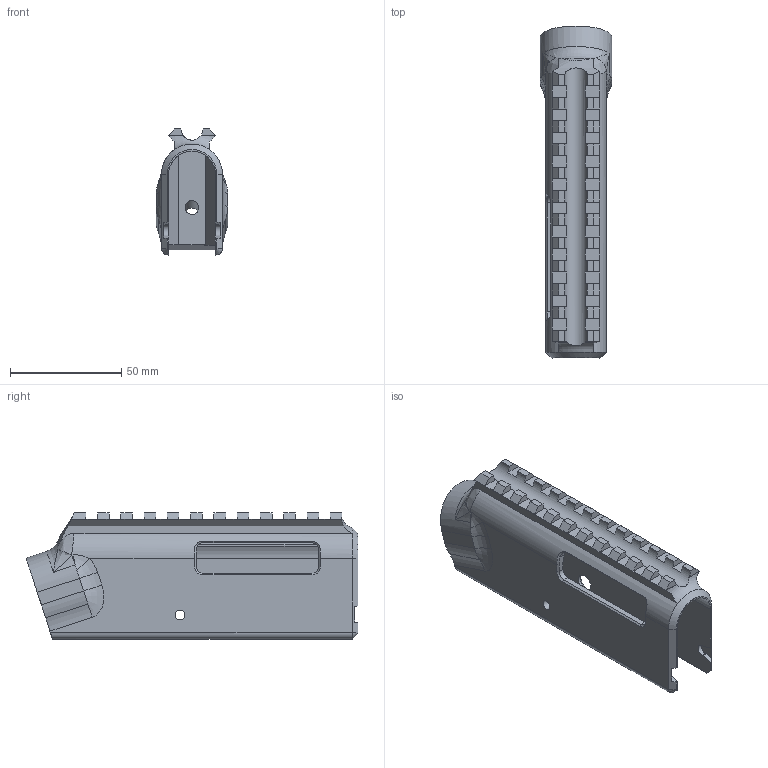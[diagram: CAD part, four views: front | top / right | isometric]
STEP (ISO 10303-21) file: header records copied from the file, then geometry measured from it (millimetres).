
FILE_DESCRIPTION(/* description */ (''),/* implementation_level */ '2;1');
FILE_NAME(/* name */ 'BAR-22 + Picatinny v5.step',/* time_stamp */ '2022-04-09T15:57:34-04:00',/* author */ (''),/* organization */ (''),/* preprocessor_version */ 'ST-DEVELOPER v18.1',/* originating_system */ 'Autodesk Translation Framework v10.14.0.1471',/* authorisation */ '');
FILE_SCHEMA (('AUTOMOTIVE_DESIGN { 1 0 10303 214 3 1 1 }'));
Length unit declared in the file: millimetre
Products named in the file (1): BAR-22 + Picatinny
Bounding box: 32.32 x 149.21 x 56.67 mm (x, y, z)
Volume: 66711.9 mm3; surface area: 35892.1 mm2
Topology: 1 solids, 1 shells, 230 faces, 626 edges, 394 vertices
Faces by surface type: plane 167, cylinder 26, bspline 23, cone 8, torus 6
Full cylindrical faces by diameter (mm): 4.35 x1, 6 x1, 7.85 x1, 21.6 x1
Entity records: 8443 total; most frequent: CARTESIAN_POINT 2715, ORIENTED_EDGE 1244, DIRECTION 1104, EDGE_CURVE 622, LINE 434, VECTOR 434, VERTEX_POINT 394, AXIS2_PLACEMENT_3D 335
